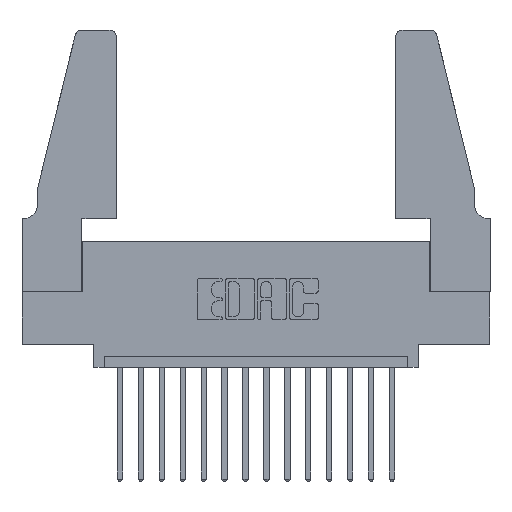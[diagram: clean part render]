
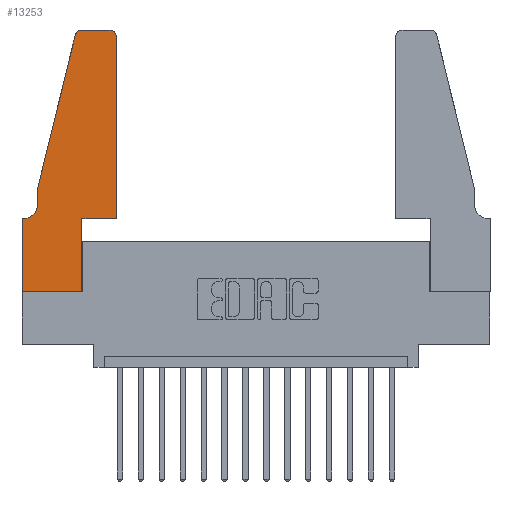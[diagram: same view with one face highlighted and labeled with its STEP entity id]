
A CAD part, top view. The second image highlights one B-rep face of the part: STEP entity #13253.
In plain terms, the highlighted planar face has unit normal (0, 0, 1).
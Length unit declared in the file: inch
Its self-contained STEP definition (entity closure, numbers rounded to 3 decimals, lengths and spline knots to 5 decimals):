
#31 = ORIENTED_EDGE ( 'NONE', *, *, #466, .T. ) ;
#134 = CARTESIAN_POINT ( 'NONE',  ( 0.4205, 1.25, 0.37 ) ) ;
#216 = CARTESIAN_POINT ( 'NONE',  ( 0.4505, 0.35, 0.37 ) ) ;
#408 = LINE ( 'NONE', #14724, #6833 ) ;
#466 = EDGE_CURVE ( 'NONE', #8561, #11666, #6301, .T. ) ;
#1228 = EDGE_CURVE ( 'NONE', #12305, #12287, #6331, .T. ) ;
#1250 = CARTESIAN_POINT ( 'NONE',  ( 0., 0., 0.37 ) ) ;
#1410 = CARTESIAN_POINT ( 'NONE',  ( 0.4505, 0.35, 0.37 ) ) ;
#1560 = EDGE_CURVE ( 'NONE', #1988, #8561, #9289, .T. ) ;
#1611 = ORIENTED_EDGE ( 'NONE', *, *, #15256, .T. ) ;
#1689 = VECTOR ( 'NONE', #10619, 39.37008 ) ;
#1695 = VECTOR ( 'NONE', #5174, 39.37008 ) ;
#1957 = VERTEX_POINT ( 'NONE', #1410 ) ;
#1988 = VERTEX_POINT ( 'NONE', #134 ) ;
#2088 = LINE ( 'NONE', #1250, #1695 ) ;
#2186 = CARTESIAN_POINT ( 'NONE',  ( 0.0755, 0.42, 0.37 ) ) ;
#2269 = DIRECTION ( 'NONE',  ( 0., -1., 0. ) ) ;
#2446 = CARTESIAN_POINT ( 'NONE',  ( 0.0055, 0.35, 0.37 ) ) ;
#2527 = CARTESIAN_POINT ( 'NONE',  ( 0.284, 1.25, 0.37 ) ) ;
#2540 = DIRECTION ( 'NONE',  ( -1., 0., 0. ) ) ;
#2739 = DIRECTION ( 'NONE',  ( 0., 1., 0. ) ) ;
#2812 = VERTEX_POINT ( 'NONE', #6526 ) ;
#3080 = DIRECTION ( 'NONE',  ( 0., 0., 1. ) ) ;
#3226 = DIRECTION ( 'NONE',  ( 0., 1., 0. ) ) ;
#3288 = AXIS2_PLACEMENT_3D ( 'NONE', #14425, #12997, #7887 ) ;
#3413 = EDGE_CURVE ( 'NONE', #14367, #1957, #16191, .T. ) ;
#3793 = ORIENTED_EDGE ( 'NONE', *, *, #13818, .T. ) ;
#3846 = ORIENTED_EDGE ( 'NONE', *, *, #5454, .T. ) ;
#4249 = VECTOR ( 'NONE', #5867, 39.37008 ) ;
#4271 = EDGE_CURVE ( 'NONE', #14935, #14488, #8918, .T. ) ;
#5174 = DIRECTION ( 'NONE',  ( 1., 0., 0. ) ) ;
#5300 = VERTEX_POINT ( 'NONE', #13229 ) ;
#5454 = EDGE_CURVE ( 'NONE', #11666, #12305, #6446, .T. ) ;
#5500 = VECTOR ( 'NONE', #2269, 39.37008 ) ;
#5867 = DIRECTION ( 'NONE',  ( -1., 0., 0. ) ) ;
#6301 = CIRCLE ( 'NONE', #14990, 0.03 ) ;
#6331 = LINE ( 'NONE', #16397, #5500 ) ;
#6446 = LINE ( 'NONE', #8406, #16291 ) ;
#6526 = CARTESIAN_POINT ( 'NONE',  ( 0.2865, 0., 0.37 ) ) ;
#6655 = AXIS2_PLACEMENT_3D ( 'NONE', #10732, #12034, #13316 ) ;
#6673 = ORIENTED_EDGE ( 'NONE', *, *, #12110, .T. ) ;
#6778 = EDGE_CURVE ( 'NONE', #5300, #2812, #2088, .T. ) ;
#6833 = VECTOR ( 'NONE', #8366, 39.37008 ) ;
#7148 = CARTESIAN_POINT ( 'NONE',  ( 0.0755, 0.35, 0.37 ) ) ;
#7258 = DIRECTION ( 'NONE',  ( -1., 0., 0. ) ) ;
#7555 = ORIENTED_EDGE ( 'NONE', *, *, #6778, .T. ) ;
#7664 = ORIENTED_EDGE ( 'NONE', *, *, #3413, .T. ) ;
#7887 = DIRECTION ( 'NONE',  ( 1., 0., 0. ) ) ;
#8004 = AXIS2_PLACEMENT_3D ( 'NONE', #15449, #8981, #2540 ) ;
#8366 = DIRECTION ( 'NONE',  ( 0., -1., 0. ) ) ;
#8406 = CARTESIAN_POINT ( 'NONE',  ( 0.0755, 0.5, 0.37 ) ) ;
#8561 = VERTEX_POINT ( 'NONE', #2527 ) ;
#8690 = ORIENTED_EDGE ( 'NONE', *, *, #1228, .T. ) ;
#8918 = LINE ( 'NONE', #7148, #12874 ) ;
#8981 = DIRECTION ( 'NONE',  ( 0., 0., -1. ) ) ;
#9046 = LINE ( 'NONE', #10944, #12469 ) ;
#9192 = CARTESIAN_POINT ( 'NONE',  ( 0.0755, 0.5, 0.37 ) ) ;
#9289 = LINE ( 'NONE', #14767, #4249 ) ;
#9427 = CARTESIAN_POINT ( 'NONE',  ( 0.284, 1.22, 0.37 ) ) ;
#9504 = LINE ( 'NONE', #14409, #12533 ) ;
#9613 = EDGE_CURVE ( 'NONE', #2812, #14367, #9504, .T. ) ;
#9990 = ORIENTED_EDGE ( 'NONE', *, *, #10929, .T. ) ;
#10009 = CIRCLE ( 'NONE', #8004, 0.07 ) ;
#10011 = ORIENTED_EDGE ( 'NONE', *, *, #4271, .T. ) ;
#10095 = EDGE_LOOP ( 'NONE', ( #14318, #31, #3846, #8690, #6673, #10011, #9990, #7555, #13675, #7664, #1611, #3793 ) ) ;
#10590 = PLANE ( 'NONE',  #3288 ) ;
#10594 = CARTESIAN_POINT ( 'NONE',  ( 0.4505, 1.22, 0.37 ) ) ;
#10619 = DIRECTION ( 'NONE',  ( 1., 0., 0. ) ) ;
#10631 = DIRECTION ( 'NONE',  ( 1., 0., 0. ) ) ;
#10732 = CARTESIAN_POINT ( 'NONE',  ( 0.4205, 1.22, 0.37 ) ) ;
#10929 = EDGE_CURVE ( 'NONE', #14488, #5300, #408, .T. ) ;
#10944 = CARTESIAN_POINT ( 'NONE',  ( 0.4505, 0.35, 0.37 ) ) ;
#11181 = CARTESIAN_POINT ( 'NONE',  ( 0.25487, 1.22718, 0.37 ) ) ;
#11666 = VERTEX_POINT ( 'NONE', #11181 ) ;
#11712 = CARTESIAN_POINT ( 'NONE',  ( 0., 0.35, 0.37 ) ) ;
#12034 = DIRECTION ( 'NONE',  ( 0., 0., 1. ) ) ;
#12067 = DIRECTION ( 'NONE',  ( -0.239, -0.971, 0. ) ) ;
#12110 = EDGE_CURVE ( 'NONE', #12287, #14935, #10009, .T. ) ;
#12235 = VERTEX_POINT ( 'NONE', #10594 ) ;
#12287 = VERTEX_POINT ( 'NONE', #2186 ) ;
#12305 = VERTEX_POINT ( 'NONE', #9192 ) ;
#12469 = VECTOR ( 'NONE', #3226, 39.37008 ) ;
#12533 = VECTOR ( 'NONE', #2739, 39.37008 ) ;
#12874 = VECTOR ( 'NONE', #7258, 39.37008 ) ;
#12997 = DIRECTION ( 'NONE',  ( 0., 0., 1. ) ) ;
#13229 = CARTESIAN_POINT ( 'NONE',  ( 0., 0., 0.37 ) ) ;
#13253 = ADVANCED_FACE ( 'NONE', ( #14595 ), #10590, .T. ) ;
#13316 = DIRECTION ( 'NONE',  ( 1., 0., 0. ) ) ;
#13675 = ORIENTED_EDGE ( 'NONE', *, *, #9613, .T. ) ;
#13818 = EDGE_CURVE ( 'NONE', #12235, #1988, #16500, .T. ) ;
#14318 = ORIENTED_EDGE ( 'NONE', *, *, #1560, .T. ) ;
#14367 = VERTEX_POINT ( 'NONE', #15415 ) ;
#14409 = CARTESIAN_POINT ( 'NONE',  ( 0.2865, 0.35, 0.37 ) ) ;
#14425 = CARTESIAN_POINT ( 'NONE',  ( 0., 0.35, 0.37 ) ) ;
#14488 = VERTEX_POINT ( 'NONE', #11712 ) ;
#14595 = FACE_OUTER_BOUND ( 'NONE', #10095, .T. ) ;
#14724 = CARTESIAN_POINT ( 'NONE',  ( 0., 0., 0.37 ) ) ;
#14767 = CARTESIAN_POINT ( 'NONE',  ( 0.2605, 1.25, 0.37 ) ) ;
#14935 = VERTEX_POINT ( 'NONE', #2446 ) ;
#14990 = AXIS2_PLACEMENT_3D ( 'NONE', #9427, #3080, #10631 ) ;
#15256 = EDGE_CURVE ( 'NONE', #1957, #12235, #9046, .T. ) ;
#15415 = CARTESIAN_POINT ( 'NONE',  ( 0.2865, 0.35, 0.37 ) ) ;
#15449 = CARTESIAN_POINT ( 'NONE',  ( 0.0055, 0.42, 0.37 ) ) ;
#16191 = LINE ( 'NONE', #216, #1689 ) ;
#16291 = VECTOR ( 'NONE', #12067, 39.37008 ) ;
#16397 = CARTESIAN_POINT ( 'NONE',  ( 0.0755, 0.5, 0.37 ) ) ;
#16500 = CIRCLE ( 'NONE', #6655, 0.03 ) ;
